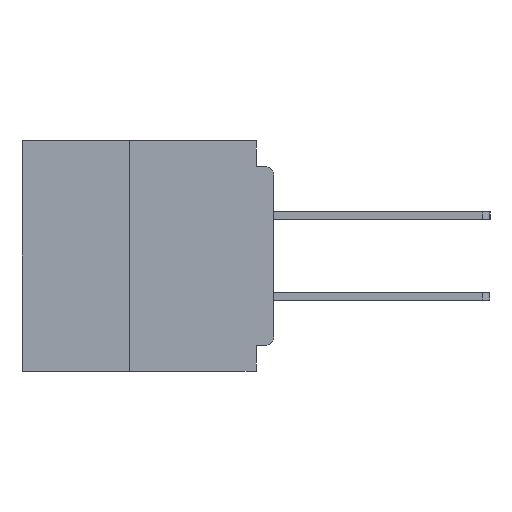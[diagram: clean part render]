
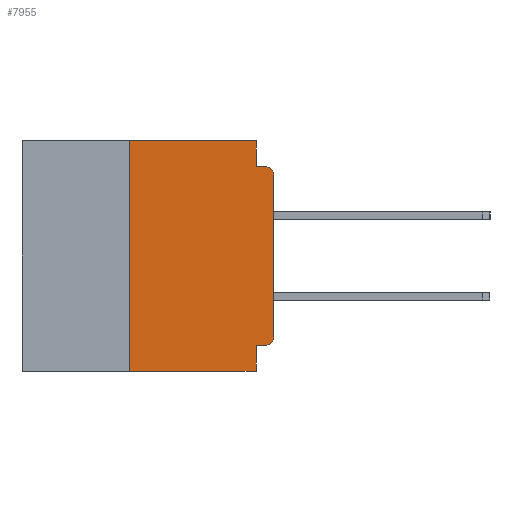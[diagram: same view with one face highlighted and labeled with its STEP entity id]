
A CAD part, left-side view. The second image highlights one B-rep face of the part: STEP entity #7955.
In plain terms, the highlighted planar face has unit normal (-1, 0, 0).
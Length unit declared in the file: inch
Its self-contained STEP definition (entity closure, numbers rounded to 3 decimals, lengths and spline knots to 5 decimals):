
#136 = ORIENTED_EDGE ( 'NONE', *, *, #27523, .F. ) ;
#2495 = VECTOR ( 'NONE', #32548, 39.37008 ) ;
#3297 = DIRECTION ( 'NONE',  ( 0., 0., -1. ) ) ;
#5834 = ORIENTED_EDGE ( 'NONE', *, *, #26785, .T. ) ;
#7265 = EDGE_CURVE ( 'NONE', #8510, #29701, #45182, .T. ) ;
#7858 = ORIENTED_EDGE ( 'NONE', *, *, #10167, .F. ) ;
#7899 = CARTESIAN_POINT ( 'NONE',  ( 0., 0.015, -0.355 ) ) ;
#7955 = ADVANCED_FACE ( 'NONE', ( #44227 ), #43427, .F. ) ;
#8510 = VERTEX_POINT ( 'NONE', #22633 ) ;
#9405 = CARTESIAN_POINT ( 'NONE',  ( 0., 0.437, -0.4 ) ) ;
#9461 = CARTESIAN_POINT ( 'NONE',  ( 0., 0., -0.06 ) ) ;
#9589 = EDGE_LOOP ( 'NONE', ( #34585, #5834, #55585, #45814, #38158, #7858, #51520, #136, #51966, #32104 ) ) ;
#9908 = VECTOR ( 'NONE', #35978, 39.37008 ) ;
#10167 = EDGE_CURVE ( 'NONE', #68032, #65991, #63081, .T. ) ;
#11386 = AXIS2_PLACEMENT_3D ( 'NONE', #54190, #22227, #59542 ) ;
#11485 = CARTESIAN_POINT ( 'NONE',  ( 0., 0.437, 0. ) ) ;
#11959 = CARTESIAN_POINT ( 'NONE',  ( 0., 0.25, 0. ) ) ;
#13814 = LINE ( 'NONE', #11485, #27979 ) ;
#14188 = VERTEX_POINT ( 'NONE', #9461 ) ;
#14885 = LINE ( 'NONE', #53277, #25724 ) ;
#14989 = CIRCLE ( 'NONE', #60414, 0.015 ) ;
#20333 = DIRECTION ( 'NONE',  ( -1., 0., 0. ) ) ;
#21551 = DIRECTION ( 'NONE',  ( 0., 0., -1. ) ) ;
#22227 = DIRECTION ( 'NONE',  ( 1., 0., 0. ) ) ;
#22633 = CARTESIAN_POINT ( 'NONE',  ( 0., 0.031, 0. ) ) ;
#22821 = CARTESIAN_POINT ( 'NONE',  ( 0., 0.031, -0.355 ) ) ;
#22883 = VERTEX_POINT ( 'NONE', #55813 ) ;
#22975 = CARTESIAN_POINT ( 'NONE',  ( 0., 0.25, -0.4 ) ) ;
#25724 = VECTOR ( 'NONE', #58637, 39.37008 ) ;
#26291 = CARTESIAN_POINT ( 'NONE',  ( 0., 0.015, -0.045 ) ) ;
#26508 = LINE ( 'NONE', #58608, #42342 ) ;
#26785 = EDGE_CURVE ( 'NONE', #14188, #67045, #14989, .T. ) ;
#27092 = AXIS2_PLACEMENT_3D ( 'NONE', #67215, #35373, #3297 ) ;
#27328 = EDGE_CURVE ( 'NONE', #68032, #28676, #38254, .T. ) ;
#27523 = EDGE_CURVE ( 'NONE', #62266, #28676, #68996, .T. ) ;
#27979 = VECTOR ( 'NONE', #48782, 39.37008 ) ;
#28676 = VERTEX_POINT ( 'NONE', #62836 ) ;
#29396 = VECTOR ( 'NONE', #32423, 39.37008 ) ;
#29701 = VERTEX_POINT ( 'NONE', #45498 ) ;
#31938 = EDGE_CURVE ( 'NONE', #29701, #67045, #14885, .T. ) ;
#32104 = ORIENTED_EDGE ( 'NONE', *, *, #36914, .T. ) ;
#32423 = DIRECTION ( 'NONE',  ( 0., 1., 0. ) ) ;
#32548 = DIRECTION ( 'NONE',  ( 0., 0., -1. ) ) ;
#33412 = EDGE_CURVE ( 'NONE', #65991, #8510, #13814, .T. ) ;
#34585 = ORIENTED_EDGE ( 'NONE', *, *, #61024, .T. ) ;
#35373 = DIRECTION ( 'NONE',  ( -1., 0., 0. ) ) ;
#35978 = DIRECTION ( 'NONE',  ( 0., -1., 0. ) ) ;
#36914 = EDGE_CURVE ( 'NONE', #56594, #22883, #42452, .T. ) ;
#38158 = ORIENTED_EDGE ( 'NONE', *, *, #33412, .F. ) ;
#38254 = LINE ( 'NONE', #9405, #9908 ) ;
#42342 = VECTOR ( 'NONE', #42497, 39.37008 ) ;
#42452 = CIRCLE ( 'NONE', #27092, 0.015 ) ;
#42497 = DIRECTION ( 'NONE',  ( 0., 0., 1. ) ) ;
#43427 = PLANE ( 'NONE',  #11386 ) ;
#43564 = LINE ( 'NONE', #53691, #29396 ) ;
#44227 = FACE_OUTER_BOUND ( 'NONE', #9589, .T. ) ;
#45182 = LINE ( 'NONE', #54037, #2495 ) ;
#45498 = CARTESIAN_POINT ( 'NONE',  ( 0., 0.031, -0.045 ) ) ;
#45814 = ORIENTED_EDGE ( 'NONE', *, *, #7265, .F. ) ;
#48782 = DIRECTION ( 'NONE',  ( 0., -1., 0. ) ) ;
#49535 = DIRECTION ( 'NONE',  ( 0., 0., 1. ) ) ;
#51520 = ORIENTED_EDGE ( 'NONE', *, *, #27328, .T. ) ;
#51966 = ORIENTED_EDGE ( 'NONE', *, *, #56309, .F. ) ;
#52258 = CARTESIAN_POINT ( 'NONE',  ( 0., 0.015, -0.06 ) ) ;
#53277 = CARTESIAN_POINT ( 'NONE',  ( 0., 0., -0.045 ) ) ;
#53287 = VECTOR ( 'NONE', #21551, 39.37008 ) ;
#53691 = CARTESIAN_POINT ( 'NONE',  ( 0., 0., -0.355 ) ) ;
#54037 = CARTESIAN_POINT ( 'NONE',  ( 0., 0.031, 0. ) ) ;
#54190 = CARTESIAN_POINT ( 'NONE',  ( 0., 0.437, 0. ) ) ;
#55585 = ORIENTED_EDGE ( 'NONE', *, *, #31938, .F. ) ;
#55813 = CARTESIAN_POINT ( 'NONE',  ( 0., 0., -0.34 ) ) ;
#56309 = EDGE_CURVE ( 'NONE', #56594, #62266, #43564, .T. ) ;
#56594 = VERTEX_POINT ( 'NONE', #7899 ) ;
#57648 = DIRECTION ( 'NONE',  ( 0., 0., -1. ) ) ;
#58119 = VECTOR ( 'NONE', #49535, 39.37008 ) ;
#58608 = CARTESIAN_POINT ( 'NONE',  ( 0., 0., 0. ) ) ;
#58637 = DIRECTION ( 'NONE',  ( 0., -1., 0. ) ) ;
#59542 = DIRECTION ( 'NONE',  ( 0., 0., -1. ) ) ;
#60414 = AXIS2_PLACEMENT_3D ( 'NONE', #52258, #20333, #57648 ) ;
#61024 = EDGE_CURVE ( 'NONE', #22883, #14188, #26508, .T. ) ;
#62266 = VERTEX_POINT ( 'NONE', #22821 ) ;
#62836 = CARTESIAN_POINT ( 'NONE',  ( 0., 0.031, -0.4 ) ) ;
#63081 = LINE ( 'NONE', #22975, #58119 ) ;
#63890 = CARTESIAN_POINT ( 'NONE',  ( 0., 0.031, -0.4 ) ) ;
#65991 = VERTEX_POINT ( 'NONE', #11959 ) ;
#66413 = CARTESIAN_POINT ( 'NONE',  ( 0., 0.25, -0.4 ) ) ;
#67045 = VERTEX_POINT ( 'NONE', #26291 ) ;
#67215 = CARTESIAN_POINT ( 'NONE',  ( 0., 0.015, -0.34 ) ) ;
#68032 = VERTEX_POINT ( 'NONE', #66413 ) ;
#68996 = LINE ( 'NONE', #63890, #53287 ) ;
